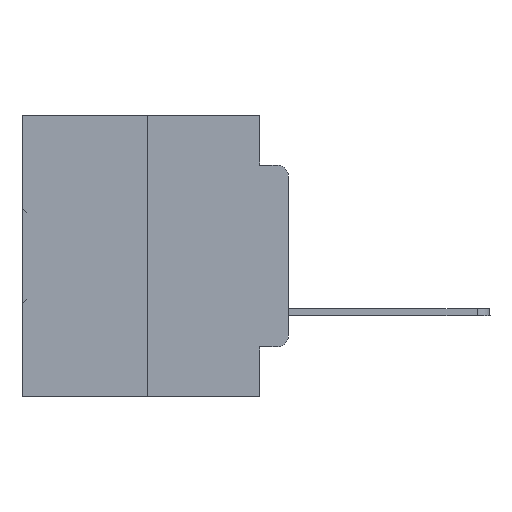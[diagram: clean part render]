
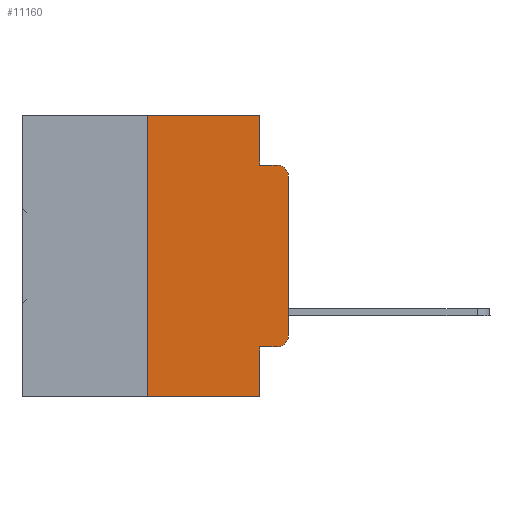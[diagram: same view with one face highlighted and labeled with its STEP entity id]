
A CAD part, left-side view. The second image highlights one B-rep face of the part: STEP entity #11160.
In plain terms, the highlighted planar face has unit normal (-1, 0, 0).
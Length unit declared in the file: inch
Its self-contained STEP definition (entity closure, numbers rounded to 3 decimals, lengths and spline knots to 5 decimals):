
#217 = EDGE_CURVE ( 'NONE', #11752, #10772, #26081, .T. ) ;
#398 = DIRECTION ( 'NONE',  ( 0., -1., 0. ) ) ;
#503 = EDGE_CURVE ( 'NONE', #17860, #1580, #10826, .T. ) ;
#687 = CARTESIAN_POINT ( 'NONE',  ( 0., 0.02, -0.1085 ) ) ;
#693 = CARTESIAN_POINT ( 'NONE',  ( 0., 0.051, 0. ) ) ;
#978 = EDGE_CURVE ( 'NONE', #2103, #27108, #4494, .T. ) ;
#1580 = VERTEX_POINT ( 'NONE', #30037 ) ;
#1655 = AXIS2_PLACEMENT_3D ( 'NONE', #687, #27470, #13996 ) ;
#1998 = DIRECTION ( 'NONE',  ( 0., -1., 0. ) ) ;
#2103 = VERTEX_POINT ( 'NONE', #15700 ) ;
#2699 = AXIS2_PLACEMENT_3D ( 'NONE', #32491, #8160, #27068 ) ;
#2881 = ORIENTED_EDGE ( 'NONE', *, *, #30594, .F. ) ;
#3393 = CARTESIAN_POINT ( 'NONE',  ( 0., 0.051, 0. ) ) ;
#4494 = CIRCLE ( 'NONE', #2699, 0.02 ) ;
#4526 = LINE ( 'NONE', #3393, #18034 ) ;
#4828 = ORIENTED_EDGE ( 'NONE', *, *, #978, .T. ) ;
#6050 = ORIENTED_EDGE ( 'NONE', *, *, #14663, .T. ) ;
#6165 = DIRECTION ( 'NONE',  ( 0., 0., -1. ) ) ;
#6443 = VECTOR ( 'NONE', #26595, 39.37008 ) ;
#7600 = CIRCLE ( 'NONE', #1655, 0.02 ) ;
#8098 = CARTESIAN_POINT ( 'NONE',  ( 0., 0.473, -0.5 ) ) ;
#8160 = DIRECTION ( 'NONE',  ( -1., 0., 0. ) ) ;
#8541 = CARTESIAN_POINT ( 'NONE',  ( 0., 0., -0.1085 ) ) ;
#9155 = CARTESIAN_POINT ( 'NONE',  ( 0., 0.473, 0. ) ) ;
#9352 = VECTOR ( 'NONE', #9845, 39.37008 ) ;
#9731 = CARTESIAN_POINT ( 'NONE',  ( 0., 0.473, 0. ) ) ;
#9845 = DIRECTION ( 'NONE',  ( 0., -1., 0. ) ) ;
#10272 = CARTESIAN_POINT ( 'NONE',  ( 0., 0.25, 0. ) ) ;
#10464 = ORIENTED_EDGE ( 'NONE', *, *, #26911, .T. ) ;
#10772 = VERTEX_POINT ( 'NONE', #27359 ) ;
#10826 = LINE ( 'NONE', #8098, #15100 ) ;
#10860 = CARTESIAN_POINT ( 'NONE',  ( 0., 0.051, -0.4115 ) ) ;
#11160 = ADVANCED_FACE ( 'NONE', ( #20097 ), #14365, .F. ) ;
#11244 = VECTOR ( 'NONE', #1998, 39.37008 ) ;
#11480 = VERTEX_POINT ( 'NONE', #10272 ) ;
#11752 = VERTEX_POINT ( 'NONE', #14642 ) ;
#13063 = ORIENTED_EDGE ( 'NONE', *, *, #20726, .F. ) ;
#13388 = LINE ( 'NONE', #26956, #30706 ) ;
#13614 = LINE ( 'NONE', #32009, #6443 ) ;
#13996 = DIRECTION ( 'NONE',  ( 0., 0., -1. ) ) ;
#14365 = PLANE ( 'NONE',  #18244 ) ;
#14642 = CARTESIAN_POINT ( 'NONE',  ( 0., 0.051, -0.0885 ) ) ;
#14663 = EDGE_CURVE ( 'NONE', #19052, #10772, #7600, .T. ) ;
#15100 = VECTOR ( 'NONE', #29529, 39.37008 ) ;
#15700 = CARTESIAN_POINT ( 'NONE',  ( 0., 0.02, -0.4115 ) ) ;
#16065 = DIRECTION ( 'NONE',  ( 0., 0., 1. ) ) ;
#16927 = DIRECTION ( 'NONE',  ( 0., 0., -1. ) ) ;
#17176 = EDGE_CURVE ( 'NONE', #24252, #11752, #4526, .T. ) ;
#17860 = VERTEX_POINT ( 'NONE', #18194 ) ;
#18034 = VECTOR ( 'NONE', #21922, 39.37008 ) ;
#18194 = CARTESIAN_POINT ( 'NONE',  ( 0., 0.25, -0.5 ) ) ;
#18244 = AXIS2_PLACEMENT_3D ( 'NONE', #9155, #24943, #16927 ) ;
#19030 = VECTOR ( 'NONE', #6165, 39.37008 ) ;
#19052 = VERTEX_POINT ( 'NONE', #8541 ) ;
#19718 = EDGE_LOOP ( 'NONE', ( #10464, #6050, #24314, #21445, #13063, #2881, #24373, #29302, #22944, #4828 ) ) ;
#20097 = FACE_OUTER_BOUND ( 'NONE', #19718, .T. ) ;
#20726 = EDGE_CURVE ( 'NONE', #11480, #24252, #29276, .T. ) ;
#21093 = EDGE_CURVE ( 'NONE', #32772, #2103, #30898, .T. ) ;
#21445 = ORIENTED_EDGE ( 'NONE', *, *, #17176, .F. ) ;
#21864 = CARTESIAN_POINT ( 'NONE',  ( 0., 0.051, 0. ) ) ;
#21922 = DIRECTION ( 'NONE',  ( 0., 0., -1. ) ) ;
#22944 = ORIENTED_EDGE ( 'NONE', *, *, #21093, .T. ) ;
#23455 = CARTESIAN_POINT ( 'NONE',  ( 0., 0.051, -0.0885 ) ) ;
#24252 = VERTEX_POINT ( 'NONE', #693 ) ;
#24314 = ORIENTED_EDGE ( 'NONE', *, *, #217, .F. ) ;
#24373 = ORIENTED_EDGE ( 'NONE', *, *, #503, .T. ) ;
#24479 = LINE ( 'NONE', #21864, #19030 ) ;
#24943 = DIRECTION ( 'NONE',  ( 1., 0., 0. ) ) ;
#26081 = LINE ( 'NONE', #23455, #11244 ) ;
#26595 = DIRECTION ( 'NONE',  ( 0., 0., 1. ) ) ;
#26911 = EDGE_CURVE ( 'NONE', #27108, #19052, #13614, .T. ) ;
#26956 = CARTESIAN_POINT ( 'NONE',  ( 0., 0.25, 0. ) ) ;
#27068 = DIRECTION ( 'NONE',  ( 0., 0., -1. ) ) ;
#27108 = VERTEX_POINT ( 'NONE', #27836 ) ;
#27359 = CARTESIAN_POINT ( 'NONE',  ( 0., 0.02, -0.0885 ) ) ;
#27470 = DIRECTION ( 'NONE',  ( -1., 0., 0. ) ) ;
#27496 = EDGE_CURVE ( 'NONE', #32772, #1580, #24479, .T. ) ;
#27836 = CARTESIAN_POINT ( 'NONE',  ( 0., 0., -0.3915 ) ) ;
#29276 = LINE ( 'NONE', #9731, #9352 ) ;
#29302 = ORIENTED_EDGE ( 'NONE', *, *, #27496, .F. ) ;
#29529 = DIRECTION ( 'NONE',  ( 0., -1., 0. ) ) ;
#30037 = CARTESIAN_POINT ( 'NONE',  ( 0., 0.051, -0.5 ) ) ;
#30594 = EDGE_CURVE ( 'NONE', #17860, #11480, #13388, .T. ) ;
#30706 = VECTOR ( 'NONE', #16065, 39.37008 ) ;
#30898 = LINE ( 'NONE', #10860, #32560 ) ;
#32009 = CARTESIAN_POINT ( 'NONE',  ( 0., 0., 0. ) ) ;
#32491 = CARTESIAN_POINT ( 'NONE',  ( 0., 0.02, -0.3915 ) ) ;
#32560 = VECTOR ( 'NONE', #398, 39.37008 ) ;
#32772 = VERTEX_POINT ( 'NONE', #34124 ) ;
#34124 = CARTESIAN_POINT ( 'NONE',  ( 0., 0.051, -0.4115 ) ) ;
